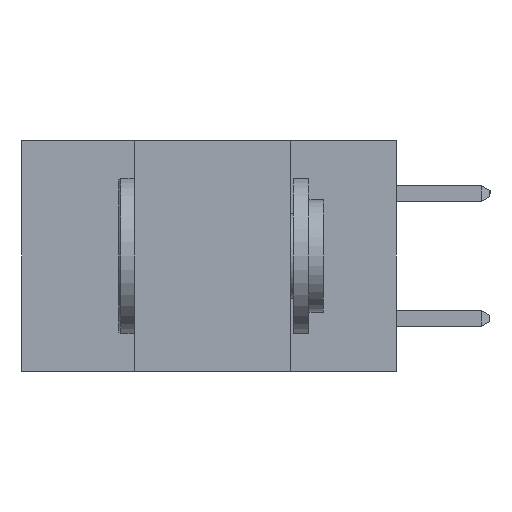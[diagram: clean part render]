
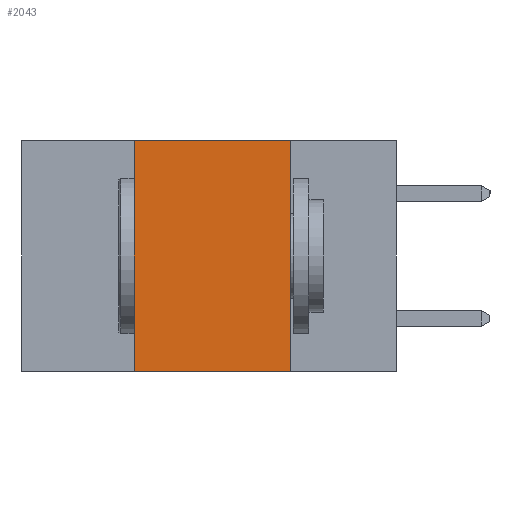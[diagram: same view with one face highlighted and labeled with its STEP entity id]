
A CAD part, left-side view. The second image highlights one B-rep face of the part: STEP entity #2043.
In plain terms, the highlighted planar face has unit normal (-1, 0, 0).
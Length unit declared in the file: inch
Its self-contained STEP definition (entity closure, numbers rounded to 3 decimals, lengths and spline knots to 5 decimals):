
#183 = VECTOR ( 'NONE', #9289, 39.37008 ) ;
#369 = CARTESIAN_POINT ( 'NONE',  ( 0., 0.17, -0.37 ) ) ;
#1106 = CARTESIAN_POINT ( 'NONE',  ( 0., 0.6, 0. ) ) ;
#1507 = EDGE_CURVE ( 'NONE', #14871, #10405, #16046, .T. ) ;
#2043 = ADVANCED_FACE ( 'NONE', ( #5218 ), #16535, .F. ) ;
#3792 = CARTESIAN_POINT ( 'NONE',  ( 0., 0.17, -0.37 ) ) ;
#3824 = ORIENTED_EDGE ( 'NONE', *, *, #12646, .T. ) ;
#4075 = CARTESIAN_POINT ( 'NONE',  ( 0., 0.6, 0. ) ) ;
#5148 = CARTESIAN_POINT ( 'NONE',  ( 0., 0.6, -0.37 ) ) ;
#5218 = FACE_OUTER_BOUND ( 'NONE', #6429, .T. ) ;
#5767 = VERTEX_POINT ( 'NONE', #3792 ) ;
#5898 = CARTESIAN_POINT ( 'NONE',  ( 0., 0.42, 0. ) ) ;
#6429 = EDGE_LOOP ( 'NONE', ( #15335, #15919, #12933, #3824 ) ) ;
#6646 = AXIS2_PLACEMENT_3D ( 'NONE', #1106, #15432, #10074 ) ;
#6874 = DIRECTION ( 'NONE',  ( 0., 0., -1. ) ) ;
#7510 = VECTOR ( 'NONE', #6874, 39.37008 ) ;
#7778 = LINE ( 'NONE', #4075, #183 ) ;
#8508 = DIRECTION ( 'NONE',  ( 0., 0., 1. ) ) ;
#8924 = DIRECTION ( 'NONE',  ( 0., -1., 0. ) ) ;
#9289 = DIRECTION ( 'NONE',  ( 0., -1., 0. ) ) ;
#10074 = DIRECTION ( 'NONE',  ( 0., 0., -1. ) ) ;
#10405 = VERTEX_POINT ( 'NONE', #5898 ) ;
#11388 = CARTESIAN_POINT ( 'NONE',  ( 0., 0.17, 0. ) ) ;
#11647 = EDGE_CURVE ( 'NONE', #10405, #15678, #7778, .T. ) ;
#11829 = LINE ( 'NONE', #369, #7510 ) ;
#12646 = EDGE_CURVE ( 'NONE', #14871, #5767, #15516, .T. ) ;
#12770 = EDGE_CURVE ( 'NONE', #15678, #5767, #11829, .T. ) ;
#12933 = ORIENTED_EDGE ( 'NONE', *, *, #1507, .F. ) ;
#13694 = CARTESIAN_POINT ( 'NONE',  ( 0., 0.42, -0.37 ) ) ;
#14472 = VECTOR ( 'NONE', #8924, 39.37008 ) ;
#14871 = VERTEX_POINT ( 'NONE', #15074 ) ;
#15074 = CARTESIAN_POINT ( 'NONE',  ( 0., 0.42, -0.37 ) ) ;
#15335 = ORIENTED_EDGE ( 'NONE', *, *, #12770, .F. ) ;
#15432 = DIRECTION ( 'NONE',  ( 1., 0., 0. ) ) ;
#15516 = LINE ( 'NONE', #5148, #14472 ) ;
#15678 = VERTEX_POINT ( 'NONE', #11388 ) ;
#15919 = ORIENTED_EDGE ( 'NONE', *, *, #11647, .F. ) ;
#16032 = VECTOR ( 'NONE', #8508, 39.37008 ) ;
#16046 = LINE ( 'NONE', #13694, #16032 ) ;
#16535 = PLANE ( 'NONE',  #6646 ) ;
